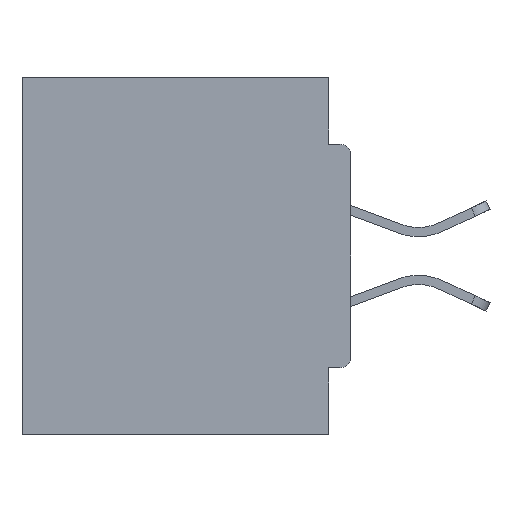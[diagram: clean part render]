
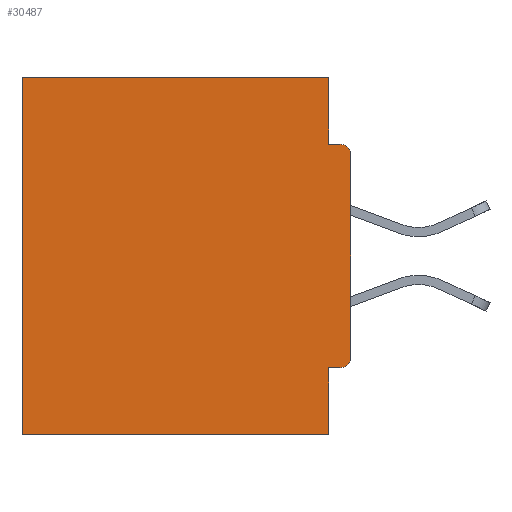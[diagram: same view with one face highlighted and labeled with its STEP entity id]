
A CAD part, left-side view. The second image highlights one B-rep face of the part: STEP entity #30487.
In plain terms, the highlighted planar face has unit normal (-1, 0, 0).
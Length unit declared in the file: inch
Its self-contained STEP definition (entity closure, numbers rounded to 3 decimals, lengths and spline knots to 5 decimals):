
#334 = ORIENTED_EDGE ( 'NONE', *, *, #17340, .F. ) ;
#783 = DIRECTION ( 'NONE',  ( 0., 0., -1. ) ) ;
#1658 = DIRECTION ( 'NONE',  ( 0., 0., -1. ) ) ;
#2539 = CARTESIAN_POINT ( 'NONE',  ( 0.298, 0., -0.5 ) ) ;
#2903 = VECTOR ( 'NONE', #10526, 39.37008 ) ;
#2938 = VERTEX_POINT ( 'NONE', #10589 ) ;
#3032 = ORIENTED_EDGE ( 'NONE', *, *, #33754, .F. ) ;
#4038 = CARTESIAN_POINT ( 'NONE',  ( 0.298, 0.015, -0.1085 ) ) ;
#4164 = DIRECTION ( 'NONE',  ( -1., 0., 0. ) ) ;
#4217 = CARTESIAN_POINT ( 'NONE',  ( 0.298, 0., 0. ) ) ;
#4901 = CARTESIAN_POINT ( 'NONE',  ( 0.298, 0.031, -0.5 ) ) ;
#4963 = EDGE_CURVE ( 'NONE', #15345, #15755, #10891, .T. ) ;
#5484 = DIRECTION ( 'NONE',  ( 0., 1., 0. ) ) ;
#6001 = LINE ( 'NONE', #4217, #27433 ) ;
#6137 = CIRCLE ( 'NONE', #21534, 0.015 ) ;
#6437 = CARTESIAN_POINT ( 'NONE',  ( 0.298, 0.031, -0.5 ) ) ;
#7083 = ORIENTED_EDGE ( 'NONE', *, *, #37275, .F. ) ;
#7591 = CARTESIAN_POINT ( 'NONE',  ( 0.298, 0.46, 0. ) ) ;
#7777 = EDGE_CURVE ( 'NONE', #30389, #24610, #26143, .T. ) ;
#8080 = LINE ( 'NONE', #2539, #35823 ) ;
#8718 = CARTESIAN_POINT ( 'NONE',  ( 0.298, 0.031, 0. ) ) ;
#9469 = CARTESIAN_POINT ( 'NONE',  ( 0.298, 0., -0.0935 ) ) ;
#9830 = VECTOR ( 'NONE', #12557, 39.37008 ) ;
#10347 = EDGE_LOOP ( 'NONE', ( #33758, #7083, #26034, #13085, #34836, #3032, #21399, #13118, #19010, #334 ) ) ;
#10364 = CARTESIAN_POINT ( 'NONE',  ( 0.298, 0., -0.3915 ) ) ;
#10526 = DIRECTION ( 'NONE',  ( 0., 1., 0. ) ) ;
#10589 = CARTESIAN_POINT ( 'NONE',  ( 0.298, 0.031, -0.0935 ) ) ;
#10891 = LINE ( 'NONE', #17088, #22747 ) ;
#10900 = CARTESIAN_POINT ( 'NONE',  ( 0.298, 0.031, -0.4065 ) ) ;
#11690 = VERTEX_POINT ( 'NONE', #20726 ) ;
#11835 = DIRECTION ( 'NONE',  ( 0., 0., -1. ) ) ;
#12098 = FACE_OUTER_BOUND ( 'NONE', #10347, .T. ) ;
#12126 = EDGE_CURVE ( 'NONE', #20827, #2938, #25674, .T. ) ;
#12557 = DIRECTION ( 'NONE',  ( 0., -1., 0. ) ) ;
#13085 = ORIENTED_EDGE ( 'NONE', *, *, #17790, .T. ) ;
#13118 = ORIENTED_EDGE ( 'NONE', *, *, #7777, .F. ) ;
#14048 = AXIS2_PLACEMENT_3D ( 'NONE', #4038, #4164, #18758 ) ;
#14637 = CARTESIAN_POINT ( 'NONE',  ( 0.298, 0.46, -0.5 ) ) ;
#14869 = LINE ( 'NONE', #9469, #9830 ) ;
#15345 = VERTEX_POINT ( 'NONE', #7591 ) ;
#15755 = VERTEX_POINT ( 'NONE', #14637 ) ;
#17088 = CARTESIAN_POINT ( 'NONE',  ( 0.298, 0.46, 0. ) ) ;
#17340 = EDGE_CURVE ( 'NONE', #11690, #37569, #36063, .T. ) ;
#17790 = EDGE_CURVE ( 'NONE', #20827, #15345, #6001, .T. ) ;
#17979 = VECTOR ( 'NONE', #36496, 39.37008 ) ;
#18758 = DIRECTION ( 'NONE',  ( 0., 0., -1. ) ) ;
#18761 = EDGE_CURVE ( 'NONE', #11690, #31023, #20578, .T. ) ;
#19010 = ORIENTED_EDGE ( 'NONE', *, *, #25386, .T. ) ;
#19082 = CARTESIAN_POINT ( 'NONE',  ( 0.298, 0., -0.4065 ) ) ;
#19156 = CARTESIAN_POINT ( 'NONE',  ( 0.298, 0.031, -0.5 ) ) ;
#20182 = DIRECTION ( 'NONE',  ( 0., 0., -1. ) ) ;
#20578 = CIRCLE ( 'NONE', #14048, 0.015 ) ;
#20726 = CARTESIAN_POINT ( 'NONE',  ( 0.298, 0., -0.1085 ) ) ;
#20827 = VERTEX_POINT ( 'NONE', #8718 ) ;
#21399 = ORIENTED_EDGE ( 'NONE', *, *, #32745, .F. ) ;
#21534 = AXIS2_PLACEMENT_3D ( 'NONE', #32269, #35303, #11835 ) ;
#22747 = VECTOR ( 'NONE', #34203, 39.37008 ) ;
#22839 = LINE ( 'NONE', #6437, #25976 ) ;
#24066 = VERTEX_POINT ( 'NONE', #4901 ) ;
#24610 = VERTEX_POINT ( 'NONE', #10900 ) ;
#24646 = DIRECTION ( 'NONE',  ( 0., 1., 0. ) ) ;
#25159 = CARTESIAN_POINT ( 'NONE',  ( 0.298, 0., 0. ) ) ;
#25386 = EDGE_CURVE ( 'NONE', #30389, #37569, #6137, .T. ) ;
#25674 = LINE ( 'NONE', #19156, #17979 ) ;
#25966 = DIRECTION ( 'NONE',  ( 1., 0., 0. ) ) ;
#25976 = VECTOR ( 'NONE', #783, 39.37008 ) ;
#26034 = ORIENTED_EDGE ( 'NONE', *, *, #12126, .F. ) ;
#26143 = LINE ( 'NONE', #19082, #2903 ) ;
#27433 = VECTOR ( 'NONE', #24646, 39.37008 ) ;
#28535 = CARTESIAN_POINT ( 'NONE',  ( 0.298, 0.015, -0.4065 ) ) ;
#28795 = CARTESIAN_POINT ( 'NONE',  ( 0.298, 0., 0. ) ) ;
#30389 = VERTEX_POINT ( 'NONE', #28535 ) ;
#30487 = ADVANCED_FACE ( 'NONE', ( #12098 ), #31797, .F. ) ;
#31023 = VERTEX_POINT ( 'NONE', #34816 ) ;
#31320 = AXIS2_PLACEMENT_3D ( 'NONE', #28795, #25966, #20182 ) ;
#31797 = PLANE ( 'NONE',  #31320 ) ;
#32269 = CARTESIAN_POINT ( 'NONE',  ( 0.298, 0.015, -0.3915 ) ) ;
#32432 = VECTOR ( 'NONE', #1658, 39.37008 ) ;
#32745 = EDGE_CURVE ( 'NONE', #24610, #24066, #22839, .T. ) ;
#33754 = EDGE_CURVE ( 'NONE', #24066, #15755, #8080, .T. ) ;
#33758 = ORIENTED_EDGE ( 'NONE', *, *, #18761, .T. ) ;
#34203 = DIRECTION ( 'NONE',  ( 0., 0., -1. ) ) ;
#34816 = CARTESIAN_POINT ( 'NONE',  ( 0.298, 0.015, -0.0935 ) ) ;
#34836 = ORIENTED_EDGE ( 'NONE', *, *, #4963, .T. ) ;
#35303 = DIRECTION ( 'NONE',  ( -1., 0., 0. ) ) ;
#35823 = VECTOR ( 'NONE', #5484, 39.37008 ) ;
#36063 = LINE ( 'NONE', #25159, #32432 ) ;
#36496 = DIRECTION ( 'NONE',  ( 0., 0., -1. ) ) ;
#37275 = EDGE_CURVE ( 'NONE', #2938, #31023, #14869, .T. ) ;
#37569 = VERTEX_POINT ( 'NONE', #10364 ) ;
